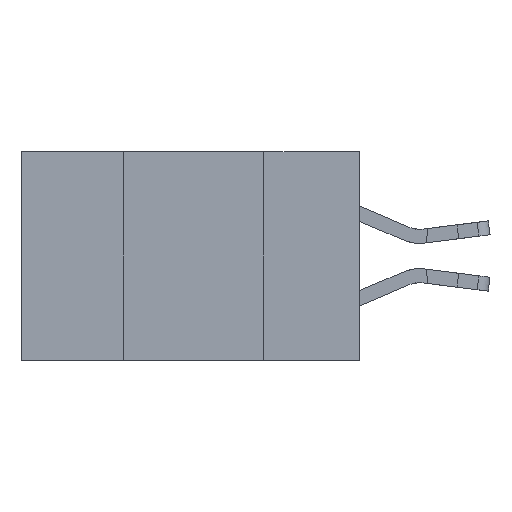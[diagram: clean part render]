
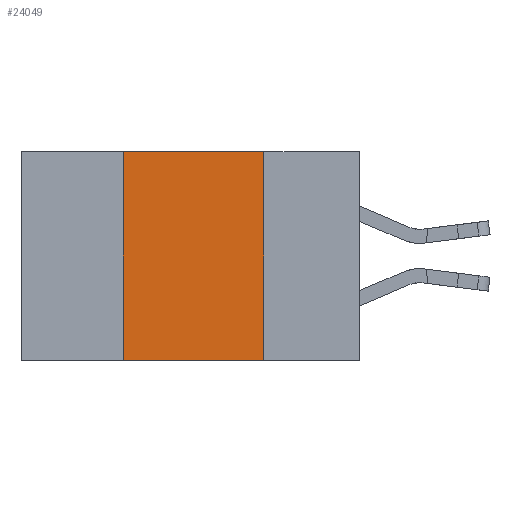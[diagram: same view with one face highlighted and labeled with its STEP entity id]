
A CAD part, left-side view. The second image highlights one B-rep face of the part: STEP entity #24049.
In plain terms, the highlighted planar face has unit normal (-1, 0, 0).
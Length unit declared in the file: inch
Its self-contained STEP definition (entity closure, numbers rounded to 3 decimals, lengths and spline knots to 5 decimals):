
#705 = CARTESIAN_POINT ( 'NONE',  ( 0., 0.17, 0. ) ) ;
#759 = AXIS2_PLACEMENT_3D ( 'NONE', #11354, #9018, #25855 ) ;
#4117 = LINE ( 'NONE', #705, #7034 ) ;
#5003 = VECTOR ( 'NONE', #12744, 39.37008 ) ;
#5248 = VERTEX_POINT ( 'NONE', #18621 ) ;
#6310 = LINE ( 'NONE', #18552, #5003 ) ;
#6426 = VERTEX_POINT ( 'NONE', #12232 ) ;
#6907 = CARTESIAN_POINT ( 'NONE',  ( 0., 0.17, -0.37 ) ) ;
#7034 = VECTOR ( 'NONE', #13090, 39.37008 ) ;
#7697 = ORIENTED_EDGE ( 'NONE', *, *, #11468, .F. ) ;
#9018 = DIRECTION ( 'NONE',  ( 1., 0., 0. ) ) ;
#10107 = EDGE_CURVE ( 'NONE', #6426, #5248, #17158, .T. ) ;
#10945 = EDGE_LOOP ( 'NONE', ( #7697, #13549, #23541, #25684 ) ) ;
#11354 = CARTESIAN_POINT ( 'NONE',  ( 0., 0.6, 0. ) ) ;
#11468 = EDGE_CURVE ( 'NONE', #15639, #22649, #4117, .T. ) ;
#12232 = CARTESIAN_POINT ( 'NONE',  ( 0., 0.42, -0.37 ) ) ;
#12744 = DIRECTION ( 'NONE',  ( 0., -1., 0. ) ) ;
#13090 = DIRECTION ( 'NONE',  ( 0., 0., -1. ) ) ;
#13549 = ORIENTED_EDGE ( 'NONE', *, *, #15656, .F. ) ;
#13705 = DIRECTION ( 'NONE',  ( 0., -1., 0. ) ) ;
#14008 = CARTESIAN_POINT ( 'NONE',  ( 0., 0.42, 0. ) ) ;
#15639 = VERTEX_POINT ( 'NONE', #20718 ) ;
#15656 = EDGE_CURVE ( 'NONE', #5248, #15639, #6310, .T. ) ;
#17158 = LINE ( 'NONE', #14008, #26217 ) ;
#18532 = VECTOR ( 'NONE', #13705, 39.37008 ) ;
#18552 = CARTESIAN_POINT ( 'NONE',  ( 0., 0.6, 0. ) ) ;
#18621 = CARTESIAN_POINT ( 'NONE',  ( 0., 0.42, 0. ) ) ;
#19079 = FACE_OUTER_BOUND ( 'NONE', #10945, .T. ) ;
#20450 = DIRECTION ( 'NONE',  ( 0., 0., 1. ) ) ;
#20718 = CARTESIAN_POINT ( 'NONE',  ( 0., 0.17, 0. ) ) ;
#21513 = PLANE ( 'NONE',  #759 ) ;
#22203 = EDGE_CURVE ( 'NONE', #6426, #22649, #24033, .T. ) ;
#22649 = VERTEX_POINT ( 'NONE', #6907 ) ;
#23541 = ORIENTED_EDGE ( 'NONE', *, *, #10107, .F. ) ;
#24033 = LINE ( 'NONE', #24143, #18532 ) ;
#24049 = ADVANCED_FACE ( 'NONE', ( #19079 ), #21513, .F. ) ;
#24143 = CARTESIAN_POINT ( 'NONE',  ( 0., 0.6, -0.37 ) ) ;
#25684 = ORIENTED_EDGE ( 'NONE', *, *, #22203, .T. ) ;
#25855 = DIRECTION ( 'NONE',  ( 0., 0., -1. ) ) ;
#26217 = VECTOR ( 'NONE', #20450, 39.37008 ) ;
